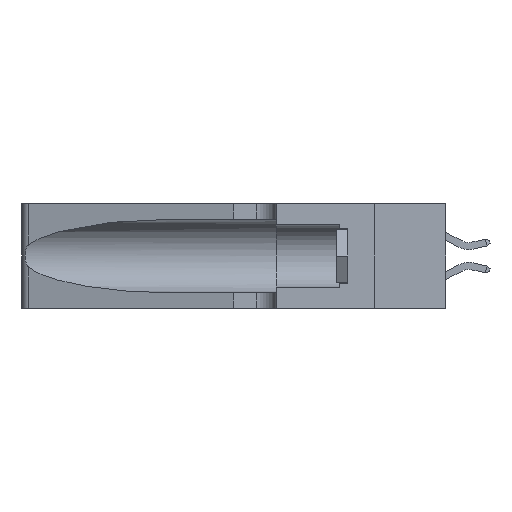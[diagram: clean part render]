
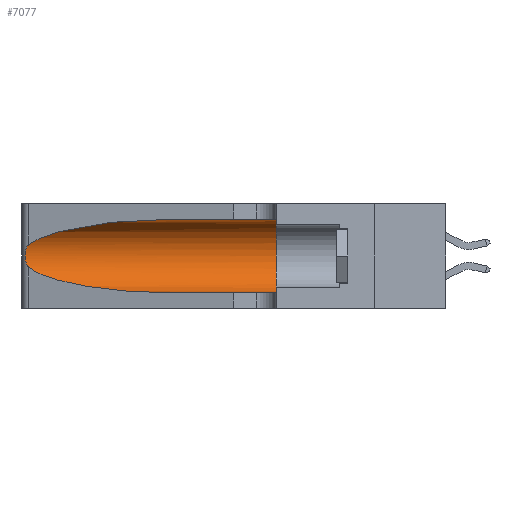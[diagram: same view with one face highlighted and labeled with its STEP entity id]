
A CAD part, left-side view. The second image highlights one B-rep face of the part: STEP entity #7077.
In plain terms, the highlighted cylindrical face has radius 3.308 mm (diameter 6.617 mm), a partial arc.
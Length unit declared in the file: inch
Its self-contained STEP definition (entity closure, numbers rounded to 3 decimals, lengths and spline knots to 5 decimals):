
#81 = DIRECTION ( 'NONE',  ( 0., -1., 0. ) ) ;
#402 = CARTESIAN_POINT ( 'NONE',  ( 0.2373, 1.15595, 0.08982 ) ) ;
#1901 = CARTESIAN_POINT ( 'NONE',  ( 0.1305, 0.72297, 0.31525 ) ) ;
#2390 = VERTEX_POINT ( 'NONE', #8842 ) ;
#2715 = CARTESIAN_POINT ( 'NONE',  ( 0.25856, 1.23593, 0.16098 ) ) ;
#3192 = DIRECTION ( 'NONE',  ( 0., 0., -1. ) ) ;
#3562 = CARTESIAN_POINT ( 'NONE',  ( 0.1305, 0.35, 0.185 ) ) ;
#5353 = CARTESIAN_POINT ( 'NONE',  ( 0.25487, 1.22718, 0.22369 ) ) ;
#5474 = CARTESIAN_POINT ( 'NONE',  ( 0.25639, 1.23186, 0.15144 ) ) ;
#6056 = CARTESIAN_POINT ( 'NONE',  ( 0.1305, 0.35, 0.05475 ) ) ;
#6218 = VECTOR ( 'NONE', #81, 39.37008 ) ;
#6257 = VERTEX_POINT ( 'NONE', #1901 ) ;
#6300 = DIRECTION ( 'NONE',  ( 0., 0., 1. ) ) ;
#7077 = ADVANCED_FACE ( 'NONE', ( #9634 ), #16088, .F. ) ;
#7079 = VERTEX_POINT ( 'NONE', #6056 ) ;
#8209 = CARTESIAN_POINT ( 'NONE',  ( 0.25487, 1.22718, 0.14631 ) ) ;
#8379 = ORIENTED_EDGE ( 'NONE', *, *, #9004, .T. ) ;
#8684 = CARTESIAN_POINT ( 'NONE',  ( 0.25487, 1.22718, 0.14631 ) ) ;
#8842 = CARTESIAN_POINT ( 'NONE',  ( 0.25487, 1.22718, 0.14631 ) ) ;
#9004 = EDGE_CURVE ( 'NONE', #12655, #2390, #9963, .T. ) ;
#9634 = FACE_OUTER_BOUND ( 'NONE', #12199, .T. ) ;
#9963 = B_SPLINE_CURVE_WITH_KNOTS ( 'NONE', 3,
 ( #5353, #21741, #10845, #29932, #13612, #32638, #16378, #33870, #19115, #2715, #21871, #5474, #24608, #8209 ),
 .UNSPECIFIED., .F., .F.,
 ( 4, 2, 2, 2, 2, 2, 4 ),
 ( 0., 0.00027, 0.00053, 0.00107, 0.0016, 0.00187, 0.00214 ),
 .UNSPECIFIED. ) ;
#10795 = CARTESIAN_POINT ( 'NONE',  ( 0.25487, 1.22718, 0.22369 ) ) ;
#10845 = CARTESIAN_POINT ( 'NONE',  ( 0.25639, 1.23184, 0.21858 ) ) ;
#12199 = EDGE_LOOP ( 'NONE', ( #30552, #8379, #22668, #29130, #33141, #14047 ) ) ;
#12655 = VERTEX_POINT ( 'NONE', #24122 ) ;
#13612 = CARTESIAN_POINT ( 'NONE',  ( 0.25854, 1.2359, 0.20912 ) ) ;
#13886 = AXIS2_PLACEMENT_3D ( 'NONE', #3562, #22697, #6300 ) ;
#14047 = ORIENTED_EDGE ( 'NONE', *, *, #20254, .F. ) ;
#14656 = CARTESIAN_POINT ( 'NONE',  ( 0.1305, 0.35, 0.31525 ) ) ;
#15586 = DIRECTION ( 'NONE',  ( 0., -1., 0. ) ) ;
#16088 = CYLINDRICAL_SURFACE ( 'NONE', #21444, 0.13025 ) ;
#16378 = CARTESIAN_POINT ( 'NONE',  ( 0.26075, 1.23896, 0.19203 ) ) ;
#16960 = CARTESIAN_POINT ( 'NONE',  ( 0.1305, 1.61858, 0.185 ) ) ;
#16964 = CARTESIAN_POINT ( 'NONE',  ( 0.1305, 0.72297, 0.05475 ) ) ;
#18935 = VECTOR ( 'NONE', #15586, 39.37008 ) ;
#18990 = EDGE_CURVE ( 'NONE', #2390, #21320, #32670, .T. ) ;
#19115 = CARTESIAN_POINT ( 'NONE',  ( 0.26017, 1.23833, 0.17102 ) ) ;
#19708 = DIRECTION ( 'NONE',  ( 0., -1., 0. ) ) ;
#20254 = EDGE_CURVE ( 'NONE', #6257, #28794, #21642, .T. ) ;
#21320 = VERTEX_POINT ( 'NONE', #34859 ) ;
#21444 = AXIS2_PLACEMENT_3D ( 'NONE', #16960, #19708, #3192 ) ;
#21642 = LINE ( 'NONE', #32806, #6218 ) ;
#21698 = CARTESIAN_POINT ( 'NONE',  ( 0.1305, 0.72297, 0.31525 ) ) ;
#21741 = CARTESIAN_POINT ( 'NONE',  ( 0.25555, 1.22994, 0.2215 ) ) ;
#21871 = CARTESIAN_POINT ( 'NONE',  ( 0.25789, 1.23486, 0.15765 ) ) ;
#22042 = EDGE_CURVE ( 'NONE', #21320, #7079, #34199, .T. ) ;
#22668 = ORIENTED_EDGE ( 'NONE', *, *, #18990, .T. ) ;
#22697 = DIRECTION ( 'NONE',  ( 0., 1., 0. ) ) ;
#23781 =( BOUNDED_CURVE ( )  B_SPLINE_CURVE ( 3, ( #21698, #35191, #27164, #10795 ),
 .UNSPECIFIED., .F., .T. ) 
 B_SPLINE_CURVE_WITH_KNOTS ( ( 4, 4 ),
 ( 1.5708, 2.84003 ),
 .UNSPECIFIED. ) 
 CURVE ( )  GEOMETRIC_REPRESENTATION_ITEM ( )  RATIONAL_B_SPLINE_CURVE ( ( 1., 0.87, 0.87, 1. ) ) 
 REPRESENTATION_ITEM ( '' )  );
#24122 = CARTESIAN_POINT ( 'NONE',  ( 0.25487, 1.22718, 0.22369 ) ) ;
#24453 = CIRCLE ( 'NONE', #13886, 0.13025 ) ;
#24608 = CARTESIAN_POINT ( 'NONE',  ( 0.25555, 1.22993, 0.14849 ) ) ;
#27164 = CARTESIAN_POINT ( 'NONE',  ( 0.2373, 1.15595, 0.28018 ) ) ;
#28794 = VERTEX_POINT ( 'NONE', #14656 ) ;
#29130 = ORIENTED_EDGE ( 'NONE', *, *, #22042, .T. ) ;
#29170 = CARTESIAN_POINT ( 'NONE',  ( 0.1305, 1.61858, 0.05475 ) ) ;
#29932 = CARTESIAN_POINT ( 'NONE',  ( 0.25787, 1.23484, 0.2124 ) ) ;
#30552 = ORIENTED_EDGE ( 'NONE', *, *, #33426, .T. ) ;
#32638 = CARTESIAN_POINT ( 'NONE',  ( 0.26018, 1.23835, 0.19895 ) ) ;
#32670 =( BOUNDED_CURVE ( )  B_SPLINE_CURVE ( 3, ( #8684, #402, #33223, #16964 ),
 .UNSPECIFIED., .F., .T. ) 
 B_SPLINE_CURVE_WITH_KNOTS ( ( 4, 4 ),
 ( 3.44316, 4.71239 ),
 .UNSPECIFIED. ) 
 CURVE ( )  GEOMETRIC_REPRESENTATION_ITEM ( )  RATIONAL_B_SPLINE_CURVE ( ( 1., 0.87, 0.87, 1. ) ) 
 REPRESENTATION_ITEM ( '' )  );
#32806 = CARTESIAN_POINT ( 'NONE',  ( 0.1305, 1.61858, 0.31525 ) ) ;
#33141 = ORIENTED_EDGE ( 'NONE', *, *, #33890, .F. ) ;
#33223 = CARTESIAN_POINT ( 'NONE',  ( 0.18966, 0.96281, 0.05475 ) ) ;
#33426 = EDGE_CURVE ( 'NONE', #6257, #12655, #23781, .T. ) ;
#33870 = CARTESIAN_POINT ( 'NONE',  ( 0.26075, 1.23896, 0.178 ) ) ;
#33890 = EDGE_CURVE ( 'NONE', #28794, #7079, #24453, .T. ) ;
#34199 = LINE ( 'NONE', #29170, #18935 ) ;
#34859 = CARTESIAN_POINT ( 'NONE',  ( 0.1305, 0.72297, 0.05475 ) ) ;
#35191 = CARTESIAN_POINT ( 'NONE',  ( 0.18966, 0.96281, 0.31525 ) ) ;
